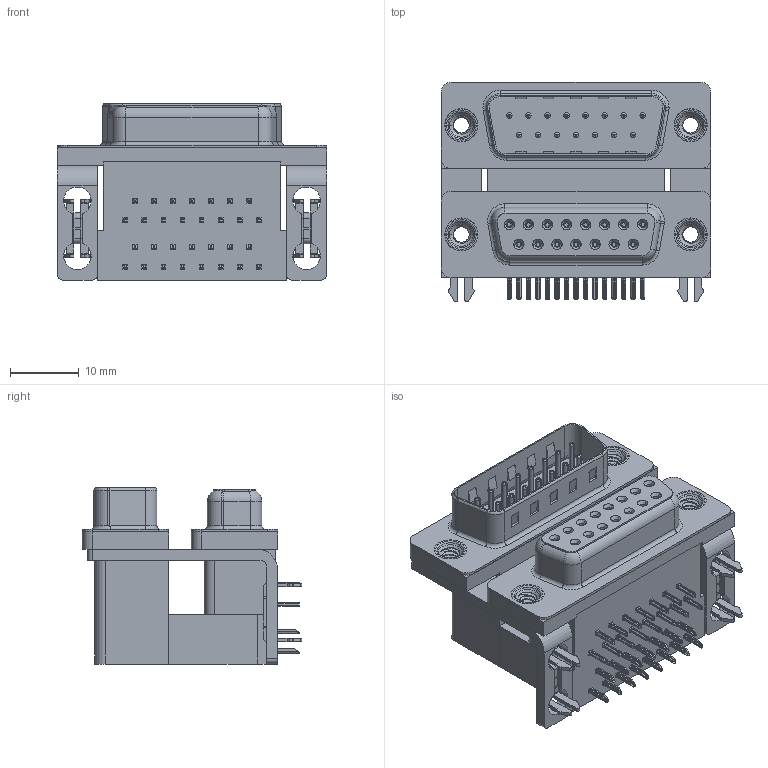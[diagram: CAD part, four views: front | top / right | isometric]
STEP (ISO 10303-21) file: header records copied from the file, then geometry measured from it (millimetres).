
FILE_DESCRIPTION (( 'STEP AP203' ), '1' );
FILE_NAME ('663-015-364-032.STEP', '2022-06-17T23:32:30', ( '' ), ( '' ), 'SwSTEP 2.0', 'SolidWorks 2020', '' );
FILE_SCHEMA (( 'CONFIG_CONTROL_DESIGN' ));
Length unit declared in the file: millimetre
Products named in the file (13): 663 Mounting Bracket_2ProngL; 663 Contact Bottom Upper_L; 663 Contact Top Upper_L; 663 2 Prong Board Lock_3; 663 Shell Receptacle_15 Contacts; 663 Shell Plug_15 Contacts; 663 Housing Lower_15 Contacts; 663-015-364-032; 663 Contact Top Lower; 663 Housing Upper_15 Contacts L; 663 Threaded Rivet_4-40; 663 Housing Spacer_15 Contacts L; 663 Contact Bottom Lower
Assembly tree (43 placements, depth 2):
  663-015-364-032
    663 Housing Lower_15 Contacts
    663 Housing Spacer_15 Contacts L
    663 Housing Upper_15 Contacts L
    663 Shell Receptacle_15 Contacts
    663 Shell Plug_15 Contacts
    663 Contact Bottom Lower  x7
    663 Contact Top Lower  x8
    663 Contact Bottom Upper_L  x7
    663 Contact Top Upper_L  x8
    663 Mounting Bracket_2ProngL  x2
    663 2 Prong Board Lock_3  x2
    663 Threaded Rivet_4-40  x4
Bounding box: 39.19 x 31.93 x 25.6 mm (x, y, z)
Volume: 14601.6 mm3; surface area: 16405.5 mm2
Topology: 43 solids, 43 shells, 4064 faces, 10485 edges, 6569 vertices
Faces by surface type: plane 2117, cylinder 1064, bspline 524, cone 200, torus 159
Entity records: 46518 total; most frequent: CARTESIAN_POINT 12336, ORIENTED_EDGE 6716, DIRECTION 6384, EDGE_CURVE 3358, LINE 2314, VECTOR 2314, VERTEX_POINT 2148, AXIS2_PLACEMENT_3D 2035
